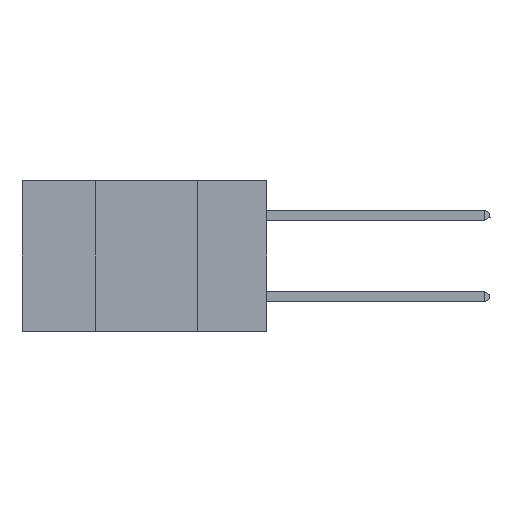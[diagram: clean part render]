
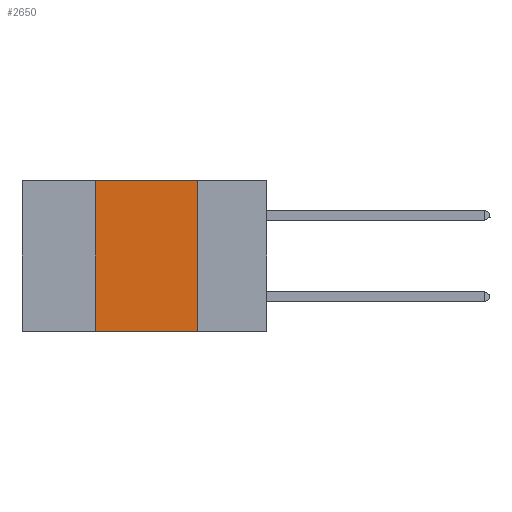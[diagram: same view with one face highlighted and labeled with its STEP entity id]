
A CAD part, left-side view. The second image highlights one B-rep face of the part: STEP entity #2650.
In plain terms, the highlighted planar face has unit normal (-1, 0, 0).
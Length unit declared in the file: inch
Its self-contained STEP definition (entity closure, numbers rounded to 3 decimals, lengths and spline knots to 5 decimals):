
#93 = AXIS2_PLACEMENT_3D ( 'NONE', #5304, #1199, #7652 ) ;
#612 = EDGE_CURVE ( 'NONE', #3180, #1455, #831, .T. ) ;
#662 = VECTOR ( 'NONE', #7711, 39.37008 ) ;
#799 = EDGE_CURVE ( 'NONE', #9438, #4849, #1909, .T. ) ;
#831 = LINE ( 'NONE', #8990, #9175 ) ;
#1092 = VECTOR ( 'NONE', #1441, 39.37008 ) ;
#1199 = DIRECTION ( 'NONE',  ( 1., 0., 0. ) ) ;
#1441 = DIRECTION ( 'NONE',  ( 0., 0., 1. ) ) ;
#1455 = VERTEX_POINT ( 'NONE', #3736 ) ;
#1909 = LINE ( 'NONE', #2822, #662 ) ;
#2650 = ADVANCED_FACE ( 'NONE', ( #5252 ), #10143, .F. ) ;
#2734 = ORIENTED_EDGE ( 'NONE', *, *, #799, .T. ) ;
#2822 = CARTESIAN_POINT ( 'NONE',  ( 0., 0.6, -0.37 ) ) ;
#3180 = VERTEX_POINT ( 'NONE', #9720 ) ;
#3228 = CARTESIAN_POINT ( 'NONE',  ( 0., 0.42, -0.37 ) ) ;
#3736 = CARTESIAN_POINT ( 'NONE',  ( 0., 0.17, 0. ) ) ;
#3867 = EDGE_CURVE ( 'NONE', #9438, #3180, #4958, .T. ) ;
#4097 = CARTESIAN_POINT ( 'NONE',  ( 0., 0.42, 0. ) ) ;
#4577 = CARTESIAN_POINT ( 'NONE',  ( 0., 0.17, -0.37 ) ) ;
#4849 = VERTEX_POINT ( 'NONE', #4577 ) ;
#4958 = LINE ( 'NONE', #4097, #1092 ) ;
#4976 = DIRECTION ( 'NONE',  ( 0., 0., -1. ) ) ;
#5226 = VECTOR ( 'NONE', #4976, 39.37008 ) ;
#5252 = FACE_OUTER_BOUND ( 'NONE', #7545, .T. ) ;
#5304 = CARTESIAN_POINT ( 'NONE',  ( 0., 0.6, 0. ) ) ;
#5358 = EDGE_CURVE ( 'NONE', #1455, #4849, #9125, .T. ) ;
#6596 = ORIENTED_EDGE ( 'NONE', *, *, #3867, .F. ) ;
#7298 = ORIENTED_EDGE ( 'NONE', *, *, #5358, .F. ) ;
#7545 = EDGE_LOOP ( 'NONE', ( #7298, #8611, #6596, #2734 ) ) ;
#7652 = DIRECTION ( 'NONE',  ( 0., 0., -1. ) ) ;
#7711 = DIRECTION ( 'NONE',  ( 0., -1., 0. ) ) ;
#8611 = ORIENTED_EDGE ( 'NONE', *, *, #612, .F. ) ;
#8990 = CARTESIAN_POINT ( 'NONE',  ( 0., 0.6, 0. ) ) ;
#9125 = LINE ( 'NONE', #10008, #5226 ) ;
#9175 = VECTOR ( 'NONE', #10705, 39.37008 ) ;
#9438 = VERTEX_POINT ( 'NONE', #3228 ) ;
#9720 = CARTESIAN_POINT ( 'NONE',  ( 0., 0.42, 0. ) ) ;
#10008 = CARTESIAN_POINT ( 'NONE',  ( 0., 0.17, 0. ) ) ;
#10143 = PLANE ( 'NONE',  #93 ) ;
#10705 = DIRECTION ( 'NONE',  ( 0., -1., 0. ) ) ;
